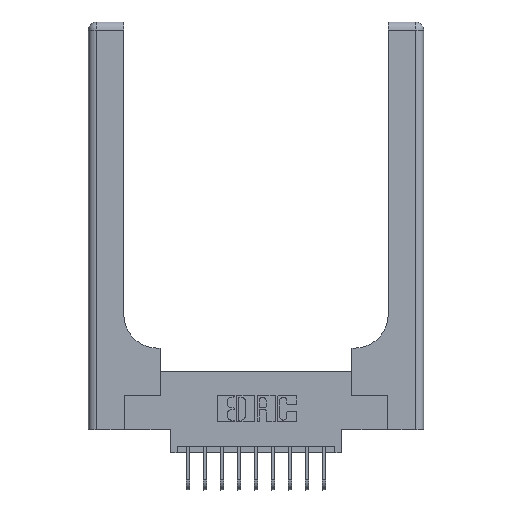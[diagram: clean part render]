
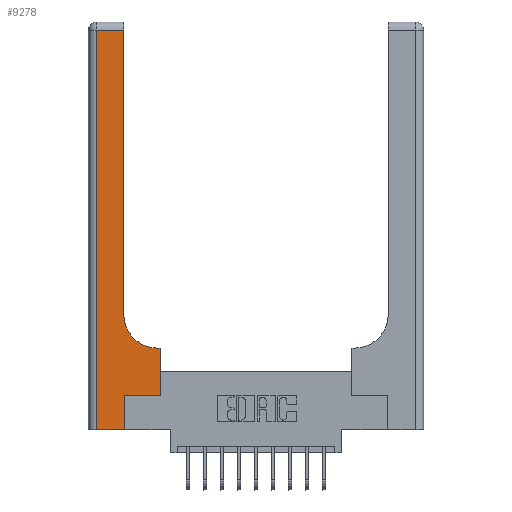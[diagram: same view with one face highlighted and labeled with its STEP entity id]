
A CAD part, top view. The second image highlights one B-rep face of the part: STEP entity #9278.
In plain terms, the highlighted planar face has unit normal (0, 0, 1).
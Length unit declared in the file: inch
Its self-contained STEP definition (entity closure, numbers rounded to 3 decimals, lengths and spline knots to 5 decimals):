
#230 = AXIS2_PLACEMENT_3D ( 'NONE', #13822, #4155, #16459 ) ;
#311 = CARTESIAN_POINT ( 'NONE',  ( 0.528, 0.25, 0.37 ) ) ;
#650 = EDGE_CURVE ( 'NONE', #16595, #13654, #4433, .T. ) ;
#666 = CARTESIAN_POINT ( 'NONE',  ( 0.26, 0.6, 0.37 ) ) ;
#1385 = EDGE_CURVE ( 'NONE', #7538, #16595, #10288, .T. ) ;
#1504 = VERTEX_POINT ( 'NONE', #5637 ) ;
#2505 = LINE ( 'NONE', #6289, #13531 ) ;
#2587 = EDGE_CURVE ( 'NONE', #5467, #16788, #6067, .T. ) ;
#2783 = VECTOR ( 'NONE', #11527, 39.37008 ) ;
#3243 = EDGE_CURVE ( 'NONE', #8332, #7538, #17712, .T. ) ;
#3251 = ORIENTED_EDGE ( 'NONE', *, *, #1385, .T. ) ;
#3632 = VECTOR ( 'NONE', #17339, 39.37008 ) ;
#4107 = CARTESIAN_POINT ( 'NONE',  ( 0.06, 0., 0.37 ) ) ;
#4155 = DIRECTION ( 'NONE',  ( 0., 0., -1. ) ) ;
#4240 = PLANE ( 'NONE',  #230 ) ;
#4433 = LINE ( 'NONE', #16742, #8771 ) ;
#5041 = VECTOR ( 'NONE', #12721, 39.37008 ) ;
#5272 = ORIENTED_EDGE ( 'NONE', *, *, #15841, .T. ) ;
#5301 = DIRECTION ( 'NONE',  ( -1., 0., 0. ) ) ;
#5467 = VERTEX_POINT ( 'NONE', #14157 ) ;
#5532 = ORIENTED_EDGE ( 'NONE', *, *, #650, .T. ) ;
#5548 = ORIENTED_EDGE ( 'NONE', *, *, #9931, .T. ) ;
#5637 = CARTESIAN_POINT ( 'NONE',  ( 0.26, 2.94, 0.37 ) ) ;
#6067 = LINE ( 'NONE', #666, #2783 ) ;
#6289 = CARTESIAN_POINT ( 'NONE',  ( 0., 2.94, 0.37 ) ) ;
#7453 = ORIENTED_EDGE ( 'NONE', *, *, #17411, .T. ) ;
#7538 = VERTEX_POINT ( 'NONE', #4107 ) ;
#8040 = ORIENTED_EDGE ( 'NONE', *, *, #14092, .T. ) ;
#8207 = CARTESIAN_POINT ( 'NONE',  ( 0.26, 3., 0.37 ) ) ;
#8332 = VERTEX_POINT ( 'NONE', #14938 ) ;
#8544 = DIRECTION ( 'NONE',  ( 1., 0., 0. ) ) ;
#8771 = VECTOR ( 'NONE', #13938, 39.37008 ) ;
#9130 = ORIENTED_EDGE ( 'NONE', *, *, #3243, .T. ) ;
#9176 = VECTOR ( 'NONE', #15298, 39.37008 ) ;
#9278 = ADVANCED_FACE ( 'NONE', ( #12388 ), #4240, .F. ) ;
#9466 = AXIS2_PLACEMENT_3D ( 'NONE', #13735, #13909, #8544 ) ;
#9770 = VECTOR ( 'NONE', #14181, 39.37008 ) ;
#9791 = EDGE_CURVE ( 'NONE', #1504, #8332, #2505, .T. ) ;
#9931 = EDGE_CURVE ( 'NONE', #12273, #5467, #10106, .T. ) ;
#10106 = LINE ( 'NONE', #14359, #9770 ) ;
#10161 = CARTESIAN_POINT ( 'NONE',  ( 0.26, 0.85, 0.37 ) ) ;
#10288 = LINE ( 'NONE', #10570, #3632 ) ;
#10570 = CARTESIAN_POINT ( 'NONE',  ( 0., 0., 0.37 ) ) ;
#11041 = LINE ( 'NONE', #8207, #9176 ) ;
#11194 = CARTESIAN_POINT ( 'NONE',  ( 0.265, 0.25, 0.37 ) ) ;
#11393 = EDGE_LOOP ( 'NONE', ( #5272, #16148, #9130, #3251, #5532, #7453, #5548, #16770, #8040 ) ) ;
#11417 = VECTOR ( 'NONE', #14852, 39.37008 ) ;
#11527 = DIRECTION ( 'NONE',  ( -1., 0., 0. ) ) ;
#12038 = CARTESIAN_POINT ( 'NONE',  ( 0.265, 0.25, 0.37 ) ) ;
#12273 = VERTEX_POINT ( 'NONE', #311 ) ;
#12388 = FACE_OUTER_BOUND ( 'NONE', #11393, .T. ) ;
#12721 = DIRECTION ( 'NONE',  ( 1., 0., 0. ) ) ;
#13531 = VECTOR ( 'NONE', #5301, 39.37008 ) ;
#13654 = VERTEX_POINT ( 'NONE', #12038 ) ;
#13735 = CARTESIAN_POINT ( 'NONE',  ( 0.51, 0.85, 0.37 ) ) ;
#13822 = CARTESIAN_POINT ( 'NONE',  ( 0., 3., 0.37 ) ) ;
#13909 = DIRECTION ( 'NONE',  ( 0., 0., -1. ) ) ;
#13938 = DIRECTION ( 'NONE',  ( 0., 1., 0. ) ) ;
#14092 = EDGE_CURVE ( 'NONE', #16788, #16247, #15653, .T. ) ;
#14157 = CARTESIAN_POINT ( 'NONE',  ( 0.528, 0.6, 0.37 ) ) ;
#14181 = DIRECTION ( 'NONE',  ( 0., 1., 0. ) ) ;
#14359 = CARTESIAN_POINT ( 'NONE',  ( 0.528, 0.25, 0.37 ) ) ;
#14483 = CARTESIAN_POINT ( 'NONE',  ( 0.51, 0.6, 0.37 ) ) ;
#14852 = DIRECTION ( 'NONE',  ( 0., -1., 0. ) ) ;
#14938 = CARTESIAN_POINT ( 'NONE',  ( 0.06, 2.94, 0.37 ) ) ;
#15298 = DIRECTION ( 'NONE',  ( 0., 1., 0. ) ) ;
#15643 = LINE ( 'NONE', #11194, #5041 ) ;
#15653 = CIRCLE ( 'NONE', #9466, 0.25 ) ;
#15841 = EDGE_CURVE ( 'NONE', #16247, #1504, #11041, .T. ) ;
#16148 = ORIENTED_EDGE ( 'NONE', *, *, #9791, .T. ) ;
#16247 = VERTEX_POINT ( 'NONE', #10161 ) ;
#16459 = DIRECTION ( 'NONE',  ( -1., 0., 0. ) ) ;
#16595 = VERTEX_POINT ( 'NONE', #16906 ) ;
#16742 = CARTESIAN_POINT ( 'NONE',  ( 0.265, 0., 0.37 ) ) ;
#16770 = ORIENTED_EDGE ( 'NONE', *, *, #2587, .T. ) ;
#16788 = VERTEX_POINT ( 'NONE', #14483 ) ;
#16906 = CARTESIAN_POINT ( 'NONE',  ( 0.265, 0., 0.37 ) ) ;
#17339 = DIRECTION ( 'NONE',  ( 1., 0., 0. ) ) ;
#17411 = EDGE_CURVE ( 'NONE', #13654, #12273, #15643, .T. ) ;
#17712 = LINE ( 'NONE', #17807, #11417 ) ;
#17807 = CARTESIAN_POINT ( 'NONE',  ( 0.06, 3., 0.37 ) ) ;
